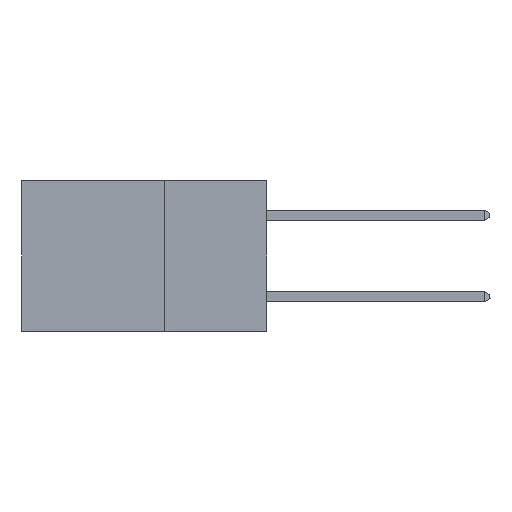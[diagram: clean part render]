
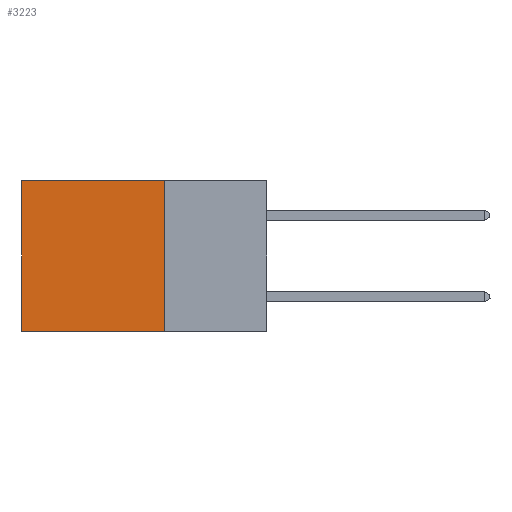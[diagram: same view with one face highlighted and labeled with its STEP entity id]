
A CAD part, left-side view. The second image highlights one B-rep face of the part: STEP entity #3223.
In plain terms, the highlighted planar face has unit normal (-1, 0, 0).
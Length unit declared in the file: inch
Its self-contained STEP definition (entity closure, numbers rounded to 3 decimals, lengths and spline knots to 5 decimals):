
#194 = VERTEX_POINT ( 'NONE', #19756 ) ;
#528 = VERTEX_POINT ( 'NONE', #20771 ) ;
#605 = DIRECTION ( 'NONE',  ( 0., 1., 0. ) ) ;
#1027 = CARTESIAN_POINT ( 'NONE',  ( 0.2875, 0.25, 0. ) ) ;
#1328 = CARTESIAN_POINT ( 'NONE',  ( 0.2875, 0.6, -0.37 ) ) ;
#1605 = DIRECTION ( 'NONE',  ( 0., 0., -1. ) ) ;
#1875 = VECTOR ( 'NONE', #14217, 39.37008 ) ;
#2305 = CARTESIAN_POINT ( 'NONE',  ( 0.2875, 0.6, 0. ) ) ;
#2933 = CARTESIAN_POINT ( 'NONE',  ( 0.2875, 0.25, 0. ) ) ;
#3223 = ADVANCED_FACE ( 'NONE', ( #18328 ), #9073, .F. ) ;
#3257 = DIRECTION ( 'NONE',  ( 1., 0., 0. ) ) ;
#5220 = EDGE_CURVE ( 'NONE', #12568, #15537, #20284, .T. ) ;
#5599 = AXIS2_PLACEMENT_3D ( 'NONE', #1027, #3257, #1605 ) ;
#6501 = VECTOR ( 'NONE', #9993, 39.37008 ) ;
#8853 = CARTESIAN_POINT ( 'NONE',  ( 0.2875, 0.25, -0.37 ) ) ;
#9073 = PLANE ( 'NONE',  #5599 ) ;
#9377 = EDGE_LOOP ( 'NONE', ( #19712, #21034, #18455, #13914 ) ) ;
#9993 = DIRECTION ( 'NONE',  ( 0., 1., 0. ) ) ;
#10348 = LINE ( 'NONE', #18338, #6501 ) ;
#10466 = DIRECTION ( 'NONE',  ( 0., 0., -1. ) ) ;
#11500 = EDGE_CURVE ( 'NONE', #194, #15537, #21147, .T. ) ;
#12568 = VERTEX_POINT ( 'NONE', #13435 ) ;
#13435 = CARTESIAN_POINT ( 'NONE',  ( 0.2875, 0.25, -0.37 ) ) ;
#13914 = ORIENTED_EDGE ( 'NONE', *, *, #15605, .T. ) ;
#14217 = DIRECTION ( 'NONE',  ( 0., 0., -1. ) ) ;
#15537 = VERTEX_POINT ( 'NONE', #1328 ) ;
#15605 = EDGE_CURVE ( 'NONE', #528, #194, #10348, .T. ) ;
#16022 = EDGE_CURVE ( 'NONE', #528, #12568, #19373, .T. ) ;
#18328 = FACE_OUTER_BOUND ( 'NONE', #9377, .T. ) ;
#18338 = CARTESIAN_POINT ( 'NONE',  ( 0.2875, 0.25, 0. ) ) ;
#18455 = ORIENTED_EDGE ( 'NONE', *, *, #16022, .F. ) ;
#19373 = LINE ( 'NONE', #2933, #1875 ) ;
#19712 = ORIENTED_EDGE ( 'NONE', *, *, #11500, .T. ) ;
#19756 = CARTESIAN_POINT ( 'NONE',  ( 0.2875, 0.6, 0. ) ) ;
#19847 = VECTOR ( 'NONE', #10466, 39.37008 ) ;
#20284 = LINE ( 'NONE', #8853, #20818 ) ;
#20771 = CARTESIAN_POINT ( 'NONE',  ( 0.2875, 0.25, 0. ) ) ;
#20818 = VECTOR ( 'NONE', #605, 39.37008 ) ;
#21034 = ORIENTED_EDGE ( 'NONE', *, *, #5220, .F. ) ;
#21147 = LINE ( 'NONE', #2305, #19847 ) ;
